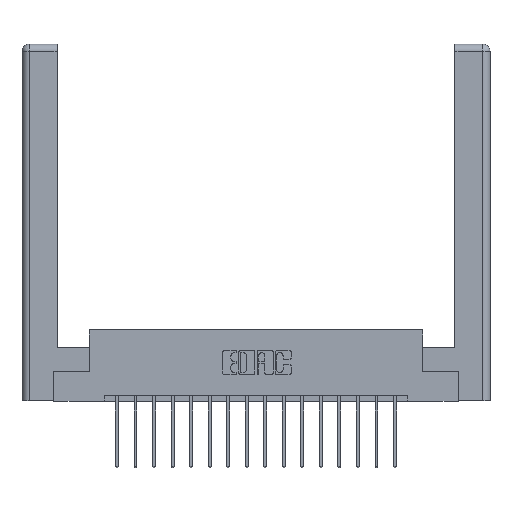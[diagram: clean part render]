
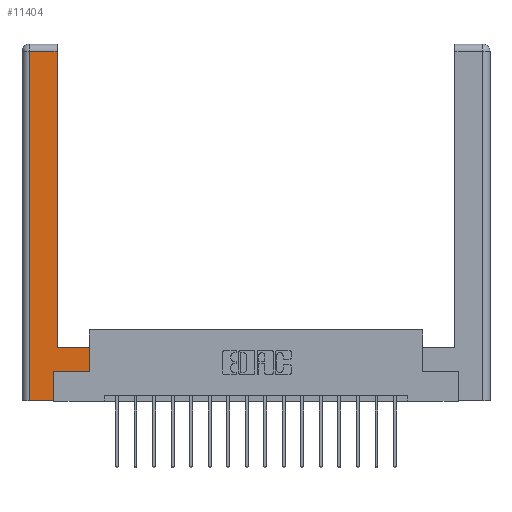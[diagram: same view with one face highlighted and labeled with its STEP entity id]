
A CAD part, top view. The second image highlights one B-rep face of the part: STEP entity #11404.
In plain terms, the highlighted planar face has unit normal (0, 0, 1).
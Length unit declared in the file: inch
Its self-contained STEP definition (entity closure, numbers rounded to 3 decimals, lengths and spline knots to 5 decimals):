
#186 = LINE ( 'NONE', #7905, #5065 ) ;
#576 = LINE ( 'NONE', #17154, #11726 ) ;
#642 = CARTESIAN_POINT ( 'NONE',  ( 0.0615, 2.94, 0. ) ) ;
#783 = VECTOR ( 'NONE', #1987, 39.37008 ) ;
#801 = DIRECTION ( 'NONE',  ( 0., -1., 0. ) ) ;
#1226 = VECTOR ( 'NONE', #12475, 39.37008 ) ;
#1583 = CARTESIAN_POINT ( 'NONE',  ( 0.565, 0.45, 0. ) ) ;
#1987 = DIRECTION ( 'NONE',  ( -1., 0., 0. ) ) ;
#2437 = CARTESIAN_POINT ( 'NONE',  ( 0.565, 0.245, 0. ) ) ;
#2898 = DIRECTION ( 'NONE',  ( -1., 0., 0. ) ) ;
#2979 = CARTESIAN_POINT ( 'NONE',  ( 0.265, 0.245, 0. ) ) ;
#3008 = EDGE_CURVE ( 'NONE', #12195, #17329, #9500, .T. ) ;
#3067 = DIRECTION ( 'NONE',  ( 0., 0., -1. ) ) ;
#3251 = CARTESIAN_POINT ( 'NONE',  ( 0.0615, 2.94, 0. ) ) ;
#3298 = EDGE_CURVE ( 'NONE', #17092, #8288, #576, .T. ) ;
#3843 = ORIENTED_EDGE ( 'NONE', *, *, #14728, .T. ) ;
#3980 = PLANE ( 'NONE',  #10265 ) ;
#3997 = VERTEX_POINT ( 'NONE', #642 ) ;
#4248 = ORIENTED_EDGE ( 'NONE', *, *, #12510, .T. ) ;
#4701 = ORIENTED_EDGE ( 'NONE', *, *, #13782, .T. ) ;
#4875 = LINE ( 'NONE', #7392, #15799 ) ;
#5065 = VECTOR ( 'NONE', #801, 39.37008 ) ;
#5725 = EDGE_CURVE ( 'NONE', #6273, #12195, #16743, .T. ) ;
#5930 = DIRECTION ( 'NONE',  ( -1., 0., 0. ) ) ;
#6273 = VERTEX_POINT ( 'NONE', #7578 ) ;
#6855 = CARTESIAN_POINT ( 'NONE',  ( 0., 0., 0. ) ) ;
#7392 = CARTESIAN_POINT ( 'NONE',  ( 0.295, 3., 0. ) ) ;
#7578 = CARTESIAN_POINT ( 'NONE',  ( 0.0615, 0., 0. ) ) ;
#7905 = CARTESIAN_POINT ( 'NONE',  ( 0.0615, 0., 0. ) ) ;
#7931 = VERTEX_POINT ( 'NONE', #12938 ) ;
#8113 = CARTESIAN_POINT ( 'NONE',  ( 0.565, 0.245, 0. ) ) ;
#8288 = VERTEX_POINT ( 'NONE', #17491 ) ;
#8825 = LINE ( 'NONE', #3251, #783 ) ;
#8977 = CARTESIAN_POINT ( 'NONE',  ( 0.265, 0.245, 0. ) ) ;
#9251 = VERTEX_POINT ( 'NONE', #2437 ) ;
#9500 = LINE ( 'NONE', #2979, #13515 ) ;
#10165 = CARTESIAN_POINT ( 'NONE',  ( 0.265, 0., 0. ) ) ;
#10265 = AXIS2_PLACEMENT_3D ( 'NONE', #6855, #3067, #5930 ) ;
#11404 = ADVANCED_FACE ( 'NONE', ( #14330 ), #3980, .F. ) ;
#11726 = VECTOR ( 'NONE', #2898, 39.37008 ) ;
#12195 = VERTEX_POINT ( 'NONE', #10165 ) ;
#12475 = DIRECTION ( 'NONE',  ( 0., 1., 0. ) ) ;
#12500 = ORIENTED_EDGE ( 'NONE', *, *, #16480, .T. ) ;
#12510 = EDGE_CURVE ( 'NONE', #17329, #9251, #17396, .T. ) ;
#12814 = ORIENTED_EDGE ( 'NONE', *, *, #17928, .T. ) ;
#12928 = DIRECTION ( 'NONE',  ( 0., 1., 0. ) ) ;
#12938 = CARTESIAN_POINT ( 'NONE',  ( 0.295, 2.94, 0. ) ) ;
#13247 = LINE ( 'NONE', #15276, #1226 ) ;
#13404 = VECTOR ( 'NONE', #18184, 39.37008 ) ;
#13515 = VECTOR ( 'NONE', #12928, 39.37008 ) ;
#13782 = EDGE_CURVE ( 'NONE', #8288, #7931, #4875, .T. ) ;
#13962 = DIRECTION ( 'NONE',  ( 1., 0., 0. ) ) ;
#14330 = FACE_OUTER_BOUND ( 'NONE', #17511, .T. ) ;
#14520 = ORIENTED_EDGE ( 'NONE', *, *, #3298, .T. ) ;
#14728 = EDGE_CURVE ( 'NONE', #3997, #6273, #186, .T. ) ;
#15276 = CARTESIAN_POINT ( 'NONE',  ( 0.565, 0.45, 0. ) ) ;
#15799 = VECTOR ( 'NONE', #16055, 39.37008 ) ;
#16055 = DIRECTION ( 'NONE',  ( 0., 1., 0. ) ) ;
#16480 = EDGE_CURVE ( 'NONE', #9251, #17092, #13247, .T. ) ;
#16743 = LINE ( 'NONE', #16822, #13404 ) ;
#16822 = CARTESIAN_POINT ( 'NONE',  ( 0.265, 0., 0. ) ) ;
#17044 = ORIENTED_EDGE ( 'NONE', *, *, #5725, .T. ) ;
#17092 = VERTEX_POINT ( 'NONE', #1583 ) ;
#17154 = CARTESIAN_POINT ( 'NONE',  ( 0.295, 0.45, 0. ) ) ;
#17329 = VERTEX_POINT ( 'NONE', #8977 ) ;
#17388 = ORIENTED_EDGE ( 'NONE', *, *, #3008, .T. ) ;
#17396 = LINE ( 'NONE', #8113, #18064 ) ;
#17491 = CARTESIAN_POINT ( 'NONE',  ( 0.295, 0.45, 0. ) ) ;
#17511 = EDGE_LOOP ( 'NONE', ( #4701, #12814, #3843, #17044, #17388, #4248, #12500, #14520 ) ) ;
#17928 = EDGE_CURVE ( 'NONE', #7931, #3997, #8825, .T. ) ;
#18064 = VECTOR ( 'NONE', #13962, 39.37008 ) ;
#18184 = DIRECTION ( 'NONE',  ( 1., 0., 0. ) ) ;
